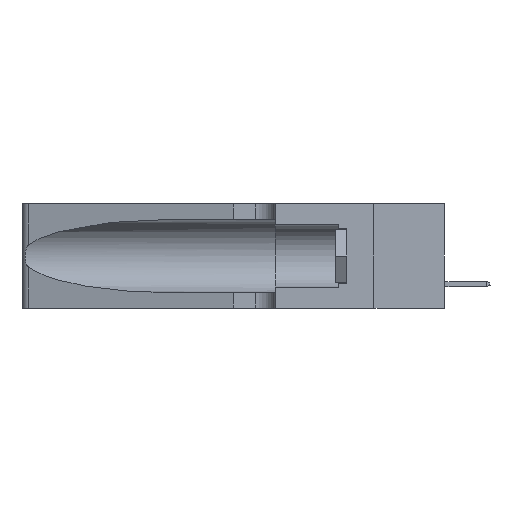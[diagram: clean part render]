
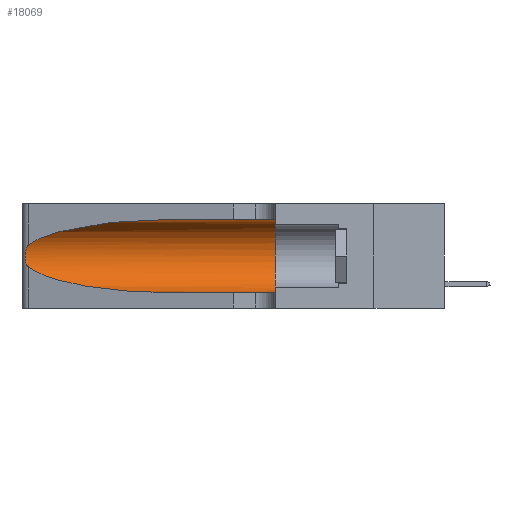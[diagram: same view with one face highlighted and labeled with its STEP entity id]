
A CAD part, left-side view. The second image highlights one B-rep face of the part: STEP entity #18069.
In plain terms, the highlighted cylindrical face has radius 3.308 mm (diameter 6.617 mm), a partial arc.
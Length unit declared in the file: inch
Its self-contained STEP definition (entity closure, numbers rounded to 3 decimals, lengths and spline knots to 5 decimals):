
#234 = CARTESIAN_POINT ( 'NONE',  ( 0.1305, 1.61858, 0.05475 ) ) ;
#1583 = EDGE_LOOP ( 'NONE', ( #2300, #7363, #3413, #17926, #3398, #30978 ) ) ;
#1700 = LINE ( 'NONE', #12458, #25124 ) ;
#1927 = CARTESIAN_POINT ( 'NONE',  ( 0.25789, 1.23486, 0.15765 ) ) ;
#2300 = ORIENTED_EDGE ( 'NONE', *, *, #16050, .T. ) ;
#2705 = VERTEX_POINT ( 'NONE', #29407 ) ;
#2812 = CARTESIAN_POINT ( 'NONE',  ( 0.2373, 1.15595, 0.08982 ) ) ;
#3398 = ORIENTED_EDGE ( 'NONE', *, *, #28169, .F. ) ;
#3413 = ORIENTED_EDGE ( 'NONE', *, *, #19267, .T. ) ;
#3438 = CARTESIAN_POINT ( 'NONE',  ( 0.1305, 0.35, 0.185 ) ) ;
#4040 = CARTESIAN_POINT ( 'NONE',  ( 0.25854, 1.2359, 0.20912 ) ) ;
#4436 = CARTESIAN_POINT ( 'NONE',  ( 0.18966, 0.96281, 0.05475 ) ) ;
#4732 = VERTEX_POINT ( 'NONE', #7105 ) ;
#5168 = DIRECTION ( 'NONE',  ( 0., -1., 0. ) ) ;
#5736 = B_SPLINE_CURVE_WITH_KNOTS ( 'NONE', 3,
 ( #30570, #16063, #11611, #23612, #4040, #16398, #13730, #8985, #13622, #25920, #1927, #11403, #20849, #28365 ),
 .UNSPECIFIED., .F., .F.,
 ( 4, 2, 2, 2, 2, 2, 4 ),
 ( 0., 0.00027, 0.00053, 0.00107, 0.0016, 0.00187, 0.00214 ),
 .UNSPECIFIED. ) ;
#6387 = CIRCLE ( 'NONE', #8951, 0.13025 ) ;
#7029 = EDGE_CURVE ( 'NONE', #19653, #4732, #28106, .T. ) ;
#7105 = CARTESIAN_POINT ( 'NONE',  ( 0.1305, 0.35, 0.05475 ) ) ;
#7363 = ORIENTED_EDGE ( 'NONE', *, *, #10875, .T. ) ;
#8072 = CARTESIAN_POINT ( 'NONE',  ( 0.25487, 1.22718, 0.14631 ) ) ;
#8775 = CARTESIAN_POINT ( 'NONE',  ( 0.1305, 0.72297, 0.05475 ) ) ;
#8951 = AXIS2_PLACEMENT_3D ( 'NONE', #3438, #10806, #27786 ) ;
#8985 = CARTESIAN_POINT ( 'NONE',  ( 0.26075, 1.23896, 0.178 ) ) ;
#9237 =( BOUNDED_CURVE ( )  B_SPLINE_CURVE ( 3, ( #25779, #16144, #20141, #29450 ),
 .UNSPECIFIED., .F., .T. ) 
 B_SPLINE_CURVE_WITH_KNOTS ( ( 4, 4 ),
 ( 1.5708, 2.84003 ),
 .UNSPECIFIED. ) 
 CURVE ( )  GEOMETRIC_REPRESENTATION_ITEM ( )  RATIONAL_B_SPLINE_CURVE ( ( 1., 0.87, 0.87, 1. ) ) 
 REPRESENTATION_ITEM ( '' )  );
#9406 = CYLINDRICAL_SURFACE ( 'NONE', #17596, 0.13025 ) ;
#10660 = CARTESIAN_POINT ( 'NONE',  ( 0.25487, 1.22718, 0.22369 ) ) ;
#10806 = DIRECTION ( 'NONE',  ( 0., 1., 0. ) ) ;
#10875 = EDGE_CURVE ( 'NONE', #19757, #19143, #5736, .T. ) ;
#11403 = CARTESIAN_POINT ( 'NONE',  ( 0.25639, 1.23186, 0.15144 ) ) ;
#11611 = CARTESIAN_POINT ( 'NONE',  ( 0.25639, 1.23184, 0.21858 ) ) ;
#12458 = CARTESIAN_POINT ( 'NONE',  ( 0.1305, 1.61858, 0.31525 ) ) ;
#13622 = CARTESIAN_POINT ( 'NONE',  ( 0.26017, 1.23833, 0.17102 ) ) ;
#13672 = DIRECTION ( 'NONE',  ( 0., 0., -1. ) ) ;
#13730 = CARTESIAN_POINT ( 'NONE',  ( 0.26075, 1.23896, 0.19203 ) ) ;
#14803 =( BOUNDED_CURVE ( )  B_SPLINE_CURVE ( 3, ( #20263, #2812, #4436, #18791 ),
 .UNSPECIFIED., .F., .T. ) 
 B_SPLINE_CURVE_WITH_KNOTS ( ( 4, 4 ),
 ( 3.44316, 4.71239 ),
 .UNSPECIFIED. ) 
 CURVE ( )  GEOMETRIC_REPRESENTATION_ITEM ( )  RATIONAL_B_SPLINE_CURVE ( ( 1., 0.87, 0.87, 1. ) ) 
 REPRESENTATION_ITEM ( '' )  );
#16050 = EDGE_CURVE ( 'NONE', #2705, #19757, #9237, .T. ) ;
#16063 = CARTESIAN_POINT ( 'NONE',  ( 0.25555, 1.22994, 0.2215 ) ) ;
#16144 = CARTESIAN_POINT ( 'NONE',  ( 0.18966, 0.96281, 0.31525 ) ) ;
#16398 = CARTESIAN_POINT ( 'NONE',  ( 0.26018, 1.23835, 0.19895 ) ) ;
#17596 = AXIS2_PLACEMENT_3D ( 'NONE', #20896, #18769, #13672 ) ;
#17887 = CARTESIAN_POINT ( 'NONE',  ( 0.1305, 0.35, 0.31525 ) ) ;
#17926 = ORIENTED_EDGE ( 'NONE', *, *, #7029, .T. ) ;
#18069 = ADVANCED_FACE ( 'NONE', ( #18103 ), #9406, .F. ) ;
#18103 = FACE_OUTER_BOUND ( 'NONE', #1583, .T. ) ;
#18769 = DIRECTION ( 'NONE',  ( 0., -1., 0. ) ) ;
#18791 = CARTESIAN_POINT ( 'NONE',  ( 0.1305, 0.72297, 0.05475 ) ) ;
#19143 = VERTEX_POINT ( 'NONE', #8072 ) ;
#19267 = EDGE_CURVE ( 'NONE', #19143, #19653, #14803, .T. ) ;
#19377 = VECTOR ( 'NONE', #19617, 39.37008 ) ;
#19617 = DIRECTION ( 'NONE',  ( 0., -1., 0. ) ) ;
#19653 = VERTEX_POINT ( 'NONE', #8775 ) ;
#19757 = VERTEX_POINT ( 'NONE', #10660 ) ;
#20141 = CARTESIAN_POINT ( 'NONE',  ( 0.2373, 1.15595, 0.28018 ) ) ;
#20263 = CARTESIAN_POINT ( 'NONE',  ( 0.25487, 1.22718, 0.14631 ) ) ;
#20849 = CARTESIAN_POINT ( 'NONE',  ( 0.25555, 1.22993, 0.14849 ) ) ;
#20896 = CARTESIAN_POINT ( 'NONE',  ( 0.1305, 1.61858, 0.185 ) ) ;
#23236 = EDGE_CURVE ( 'NONE', #2705, #24010, #1700, .T. ) ;
#23612 = CARTESIAN_POINT ( 'NONE',  ( 0.25787, 1.23484, 0.2124 ) ) ;
#24010 = VERTEX_POINT ( 'NONE', #17887 ) ;
#25124 = VECTOR ( 'NONE', #5168, 39.37008 ) ;
#25779 = CARTESIAN_POINT ( 'NONE',  ( 0.1305, 0.72297, 0.31525 ) ) ;
#25920 = CARTESIAN_POINT ( 'NONE',  ( 0.25856, 1.23593, 0.16098 ) ) ;
#27786 = DIRECTION ( 'NONE',  ( 0., 0., 1. ) ) ;
#28106 = LINE ( 'NONE', #234, #19377 ) ;
#28169 = EDGE_CURVE ( 'NONE', #24010, #4732, #6387, .T. ) ;
#28365 = CARTESIAN_POINT ( 'NONE',  ( 0.25487, 1.22718, 0.14631 ) ) ;
#29407 = CARTESIAN_POINT ( 'NONE',  ( 0.1305, 0.72297, 0.31525 ) ) ;
#29450 = CARTESIAN_POINT ( 'NONE',  ( 0.25487, 1.22718, 0.22369 ) ) ;
#30570 = CARTESIAN_POINT ( 'NONE',  ( 0.25487, 1.22718, 0.22369 ) ) ;
#30978 = ORIENTED_EDGE ( 'NONE', *, *, #23236, .F. ) ;
